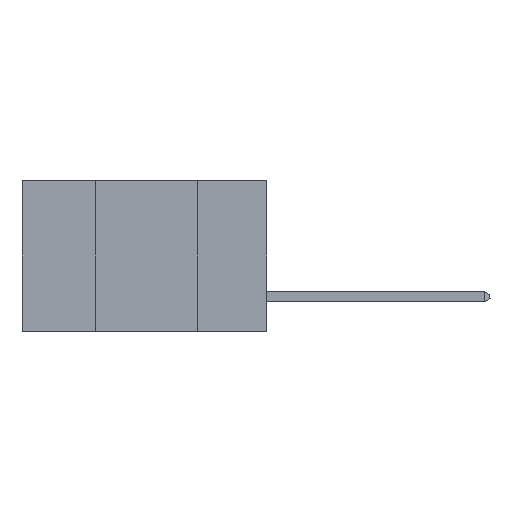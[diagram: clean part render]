
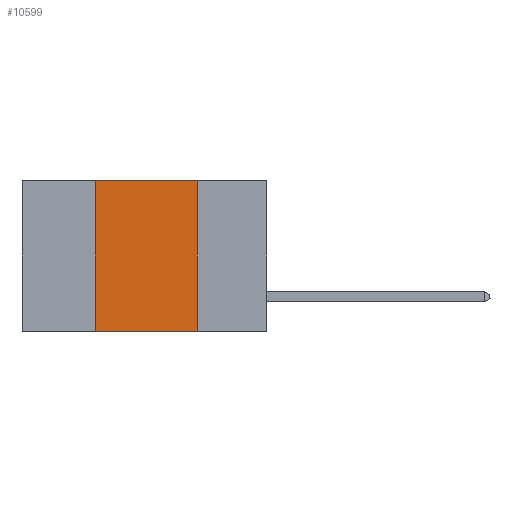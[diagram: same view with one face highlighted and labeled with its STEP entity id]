
A CAD part, left-side view. The second image highlights one B-rep face of the part: STEP entity #10599.
In plain terms, the highlighted planar face has unit normal (-1, 0, 0).
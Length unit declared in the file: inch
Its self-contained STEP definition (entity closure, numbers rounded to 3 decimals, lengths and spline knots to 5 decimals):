
#188 = CARTESIAN_POINT ( 'NONE',  ( 0., 0.17, -0.37 ) ) ;
#226 = FACE_OUTER_BOUND ( 'NONE', #7844, .T. ) ;
#651 = DIRECTION ( 'NONE',  ( 0., -1., 0. ) ) ;
#972 = DIRECTION ( 'NONE',  ( 1., 0., 0. ) ) ;
#1705 = EDGE_CURVE ( 'NONE', #7873, #2730, #10308, .T. ) ;
#1857 = VECTOR ( 'NONE', #7266, 39.37008 ) ;
#2082 = CARTESIAN_POINT ( 'NONE',  ( 0., 0.42, 0. ) ) ;
#2233 = DIRECTION ( 'NONE',  ( 0., 0., -1. ) ) ;
#2267 = DIRECTION ( 'NONE',  ( 0., 0., -1. ) ) ;
#2730 = VERTEX_POINT ( 'NONE', #188 ) ;
#3719 = LINE ( 'NONE', #7195, #8176 ) ;
#4263 = ORIENTED_EDGE ( 'NONE', *, *, #1705, .F. ) ;
#5093 = DIRECTION ( 'NONE',  ( 0., -1., 0. ) ) ;
#5751 = CARTESIAN_POINT ( 'NONE',  ( 0., 0.42, 0. ) ) ;
#5821 = ORIENTED_EDGE ( 'NONE', *, *, #9708, .F. ) ;
#6050 = VERTEX_POINT ( 'NONE', #5751 ) ;
#6672 = EDGE_CURVE ( 'NONE', #8642, #2730, #3719, .T. ) ;
#6778 = ORIENTED_EDGE ( 'NONE', *, *, #11117, .F. ) ;
#6904 = VECTOR ( 'NONE', #651, 39.37008 ) ;
#7054 = ORIENTED_EDGE ( 'NONE', *, *, #6672, .T. ) ;
#7099 = CARTESIAN_POINT ( 'NONE',  ( 0., 0.6, 0. ) ) ;
#7195 = CARTESIAN_POINT ( 'NONE',  ( 0., 0.6, -0.37 ) ) ;
#7266 = DIRECTION ( 'NONE',  ( 0., 0., 1. ) ) ;
#7844 = EDGE_LOOP ( 'NONE', ( #4263, #6778, #5821, #7054 ) ) ;
#7873 = VERTEX_POINT ( 'NONE', #9243 ) ;
#8108 = VECTOR ( 'NONE', #2233, 39.37008 ) ;
#8176 = VECTOR ( 'NONE', #5093, 39.37008 ) ;
#8642 = VERTEX_POINT ( 'NONE', #9628 ) ;
#8926 = AXIS2_PLACEMENT_3D ( 'NONE', #7099, #972, #2267 ) ;
#9243 = CARTESIAN_POINT ( 'NONE',  ( 0., 0.17, 0. ) ) ;
#9619 = LINE ( 'NONE', #11833, #6904 ) ;
#9628 = CARTESIAN_POINT ( 'NONE',  ( 0., 0.42, -0.37 ) ) ;
#9708 = EDGE_CURVE ( 'NONE', #8642, #6050, #10762, .T. ) ;
#10308 = LINE ( 'NONE', #11559, #8108 ) ;
#10599 = ADVANCED_FACE ( 'NONE', ( #226 ), #11033, .F. ) ;
#10762 = LINE ( 'NONE', #2082, #1857 ) ;
#11033 = PLANE ( 'NONE',  #8926 ) ;
#11117 = EDGE_CURVE ( 'NONE', #6050, #7873, #9619, .T. ) ;
#11559 = CARTESIAN_POINT ( 'NONE',  ( 0., 0.17, 0. ) ) ;
#11833 = CARTESIAN_POINT ( 'NONE',  ( 0., 0.6, 0. ) ) ;
